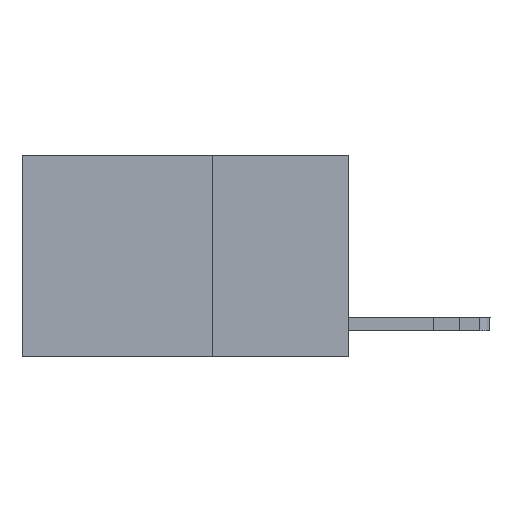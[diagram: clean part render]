
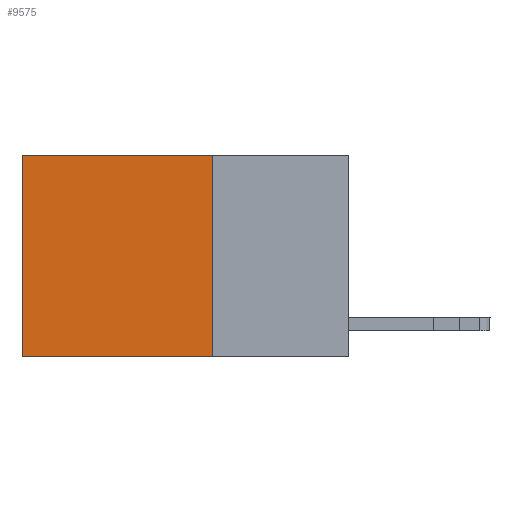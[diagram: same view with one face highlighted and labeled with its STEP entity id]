
A CAD part, left-side view. The second image highlights one B-rep face of the part: STEP entity #9575.
In plain terms, the highlighted planar face has unit normal (-1, 0, 0).
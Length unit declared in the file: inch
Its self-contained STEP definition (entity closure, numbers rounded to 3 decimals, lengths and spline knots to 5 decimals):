
#393 = VERTEX_POINT ( 'NONE', #11816 ) ;
#394 = DIRECTION ( 'NONE',  ( 0., 1., 0. ) ) ;
#678 = VERTEX_POINT ( 'NONE', #5301 ) ;
#1084 = VECTOR ( 'NONE', #7825, 39.37008 ) ;
#1317 = CARTESIAN_POINT ( 'NONE',  ( 0.2625, 0.25, 0. ) ) ;
#1428 = CARTESIAN_POINT ( 'NONE',  ( 0.2625, 0.25, -0.37 ) ) ;
#1521 = CARTESIAN_POINT ( 'NONE',  ( 0.2625, 0.6, -0.37 ) ) ;
#2254 = DIRECTION ( 'NONE',  ( 0., 0., -1. ) ) ;
#2909 = DIRECTION ( 'NONE',  ( 0., 0., -1. ) ) ;
#2955 = CARTESIAN_POINT ( 'NONE',  ( 0.2625, 0.25, 0. ) ) ;
#2997 = LINE ( 'NONE', #13305, #6503 ) ;
#3143 = FACE_OUTER_BOUND ( 'NONE', #12535, .T. ) ;
#4616 = LINE ( 'NONE', #12901, #11622 ) ;
#4728 = ORIENTED_EDGE ( 'NONE', *, *, #4730, .F. ) ;
#4730 = EDGE_CURVE ( 'NONE', #10150, #6934, #4616, .T. ) ;
#5301 = CARTESIAN_POINT ( 'NONE',  ( 0.2625, 0.6, 0. ) ) ;
#5421 = DIRECTION ( 'NONE',  ( 1., 0., 0. ) ) ;
#5463 = EDGE_CURVE ( 'NONE', #393, #10150, #12247, .T. ) ;
#6023 = LINE ( 'NONE', #13214, #10108 ) ;
#6503 = VECTOR ( 'NONE', #13372, 39.37008 ) ;
#6568 = ORIENTED_EDGE ( 'NONE', *, *, #9469, .T. ) ;
#6934 = VERTEX_POINT ( 'NONE', #1521 ) ;
#6961 = AXIS2_PLACEMENT_3D ( 'NONE', #1317, #5421, #2254 ) ;
#7825 = DIRECTION ( 'NONE',  ( 0., 0., -1. ) ) ;
#8047 = EDGE_CURVE ( 'NONE', #678, #6934, #6023, .T. ) ;
#9469 = EDGE_CURVE ( 'NONE', #393, #678, #2997, .T. ) ;
#9575 = ADVANCED_FACE ( 'NONE', ( #3143 ), #11535, .F. ) ;
#9820 = ORIENTED_EDGE ( 'NONE', *, *, #8047, .T. ) ;
#10108 = VECTOR ( 'NONE', #2909, 39.37008 ) ;
#10150 = VERTEX_POINT ( 'NONE', #1428 ) ;
#11535 = PLANE ( 'NONE',  #6961 ) ;
#11622 = VECTOR ( 'NONE', #394, 39.37008 ) ;
#11816 = CARTESIAN_POINT ( 'NONE',  ( 0.2625, 0.25, 0. ) ) ;
#12247 = LINE ( 'NONE', #2955, #1084 ) ;
#12535 = EDGE_LOOP ( 'NONE', ( #9820, #4728, #12556, #6568 ) ) ;
#12556 = ORIENTED_EDGE ( 'NONE', *, *, #5463, .F. ) ;
#12901 = CARTESIAN_POINT ( 'NONE',  ( 0.2625, 0.25, -0.37 ) ) ;
#13214 = CARTESIAN_POINT ( 'NONE',  ( 0.2625, 0.6, 0. ) ) ;
#13305 = CARTESIAN_POINT ( 'NONE',  ( 0.2625, 0.25, 0. ) ) ;
#13372 = DIRECTION ( 'NONE',  ( 0., 1., 0. ) ) ;
